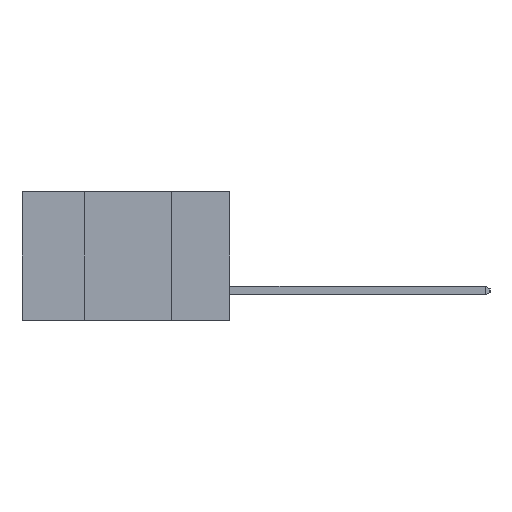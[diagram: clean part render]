
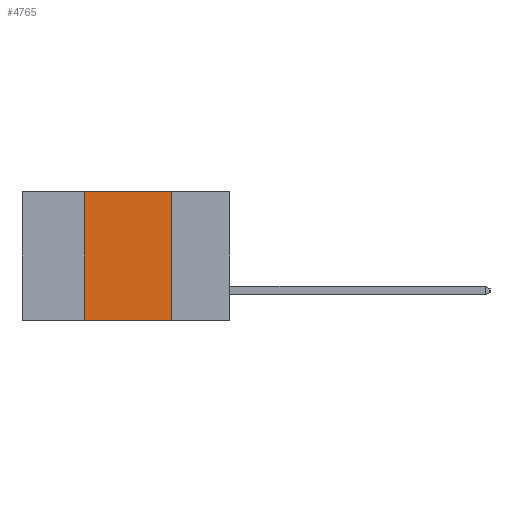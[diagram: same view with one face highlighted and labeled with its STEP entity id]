
A CAD part, left-side view. The second image highlights one B-rep face of the part: STEP entity #4765.
In plain terms, the highlighted planar face has unit normal (-1, 0, 0).
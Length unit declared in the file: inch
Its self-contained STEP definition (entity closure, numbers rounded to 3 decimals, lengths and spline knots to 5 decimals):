
#2722 = VECTOR ( 'NONE', #4658, 39.37008 ) ;
#3188 = LINE ( 'NONE', #19321, #7391 ) ;
#3895 = CARTESIAN_POINT ( 'NONE',  ( 0., 0.6, 0. ) ) ;
#4657 = EDGE_CURVE ( 'NONE', #20590, #17330, #12162, .T. ) ;
#4658 = DIRECTION ( 'NONE',  ( 0., -1., 0. ) ) ;
#4765 = ADVANCED_FACE ( 'NONE', ( #9958 ), #20743, .F. ) ;
#5120 = CARTESIAN_POINT ( 'NONE',  ( 0., 0.42, -0.37 ) ) ;
#6201 = LINE ( 'NONE', #10076, #10946 ) ;
#6403 = ORIENTED_EDGE ( 'NONE', *, *, #19640, .T. ) ;
#7229 = ORIENTED_EDGE ( 'NONE', *, *, #4657, .F. ) ;
#7391 = VECTOR ( 'NONE', #21005, 39.37008 ) ;
#9014 = VECTOR ( 'NONE', #10662, 39.37008 ) ;
#9304 = EDGE_CURVE ( 'NONE', #17330, #10782, #6201, .T. ) ;
#9485 = ORIENTED_EDGE ( 'NONE', *, *, #20770, .F. ) ;
#9958 = FACE_OUTER_BOUND ( 'NONE', #19655, .T. ) ;
#9961 = AXIS2_PLACEMENT_3D ( 'NONE', #20793, #20739, #20696 ) ;
#9973 = DIRECTION ( 'NONE',  ( 0., 0., -1. ) ) ;
#10076 = CARTESIAN_POINT ( 'NONE',  ( 0., 0.17, -0.37 ) ) ;
#10110 = LINE ( 'NONE', #14022, #9014 ) ;
#10662 = DIRECTION ( 'NONE',  ( 0., 0., 1. ) ) ;
#10782 = VERTEX_POINT ( 'NONE', #21102 ) ;
#10946 = VECTOR ( 'NONE', #9973, 39.37008 ) ;
#12162 = LINE ( 'NONE', #3895, #2722 ) ;
#14022 = CARTESIAN_POINT ( 'NONE',  ( 0., 0.42, -0.37 ) ) ;
#14875 = CARTESIAN_POINT ( 'NONE',  ( 0., 0.17, 0. ) ) ;
#16023 = ORIENTED_EDGE ( 'NONE', *, *, #9304, .F. ) ;
#17124 = VERTEX_POINT ( 'NONE', #5120 ) ;
#17330 = VERTEX_POINT ( 'NONE', #14875 ) ;
#19321 = CARTESIAN_POINT ( 'NONE',  ( 0., 0.6, -0.37 ) ) ;
#19640 = EDGE_CURVE ( 'NONE', #17124, #10782, #3188, .T. ) ;
#19655 = EDGE_LOOP ( 'NONE', ( #16023, #7229, #9485, #6403 ) ) ;
#20590 = VERTEX_POINT ( 'NONE', #22094 ) ;
#20696 = DIRECTION ( 'NONE',  ( 0., 0., -1. ) ) ;
#20739 = DIRECTION ( 'NONE',  ( 1., 0., 0. ) ) ;
#20743 = PLANE ( 'NONE',  #9961 ) ;
#20770 = EDGE_CURVE ( 'NONE', #17124, #20590, #10110, .T. ) ;
#20793 = CARTESIAN_POINT ( 'NONE',  ( 0., 0.6, 0. ) ) ;
#21005 = DIRECTION ( 'NONE',  ( 0., -1., 0. ) ) ;
#21102 = CARTESIAN_POINT ( 'NONE',  ( 0., 0.17, -0.37 ) ) ;
#22094 = CARTESIAN_POINT ( 'NONE',  ( 0., 0.42, 0. ) ) ;
